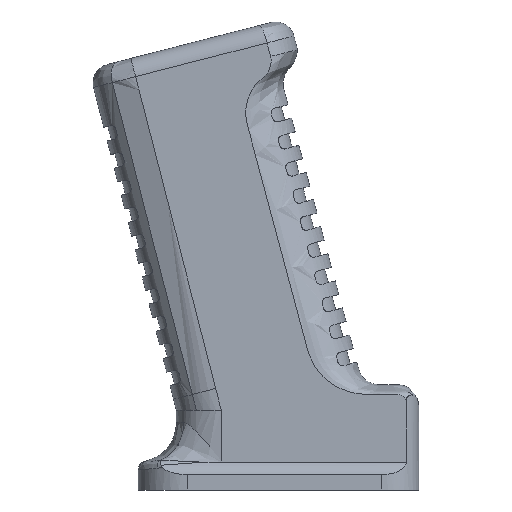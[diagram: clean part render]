
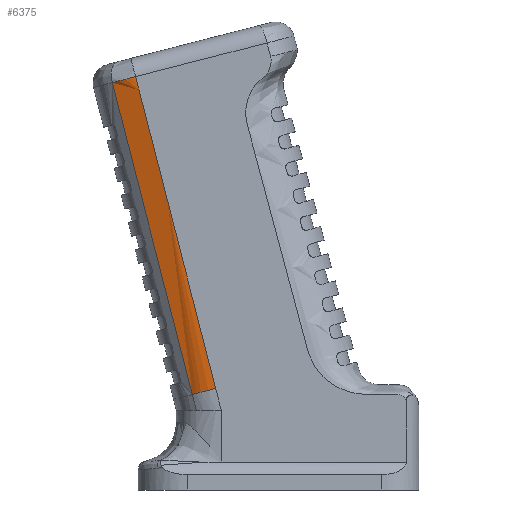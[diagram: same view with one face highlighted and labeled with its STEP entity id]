
A CAD part, front view. The second image highlights one B-rep face of the part: STEP entity #6375.
In plain terms, the highlighted free-form (B-spline) face has degree [3, 1] with [8, 2] control points.
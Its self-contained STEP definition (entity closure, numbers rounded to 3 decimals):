
#403=LINE('',#13296,#897);
#419=LINE('',#13652,#913);
#420=LINE('',#13654,#914);
#421=LINE('',#13656,#915);
#422=LINE('',#13658,#916);
#423=LINE('',#13660,#917);
#897=VECTOR('',#7216,10.);
#913=VECTOR('',#7262,10.);
#914=VECTOR('',#7263,10.);
#915=VECTOR('',#7264,10.);
#916=VECTOR('',#7265,10.);
#917=VECTOR('',#7266,10.);
#1528=FACE_OUTER_BOUND('',#1881,.T.);
#1881=EDGE_LOOP('',(#5424,#5425,#5426,#5427,#5428,#5429,#5430,#5431));
#2388=B_SPLINE_CURVE_WITH_KNOTS('',3,(#18486,#18487,#18488,#18489,#18490,
#18491),.UNSPECIFIED.,.F.,.F.,(4,2,4),(0.,0.025,0.321),
 .UNSPECIFIED.);
#2390=B_SPLINE_CURVE_WITH_KNOTS('',3,(#18559,#18560,#18561,#18562,#18563,
#18564,#18565,#18566,#18567,#18568),.UNSPECIFIED.,.F.,.F.,(4,3,3,4),(-1.549,
-1.43,-1.311,-1.28),.UNSPECIFIED.);
#2753=VERTEX_POINT('',#13281);
#2754=VERTEX_POINT('',#13295);
#2771=VERTEX_POINT('',#13649);
#2772=VERTEX_POINT('',#13651);
#2773=VERTEX_POINT('',#13653);
#2774=VERTEX_POINT('',#13655);
#2775=VERTEX_POINT('',#13657);
#2776=VERTEX_POINT('',#13659);
#3511=EDGE_CURVE('',#2753,#2754,#403,.T.);
#3546=EDGE_CURVE('',#2772,#2771,#419,.T.);
#3547=EDGE_CURVE('',#2773,#2772,#420,.T.);
#3548=EDGE_CURVE('',#2774,#2773,#421,.T.);
#3549=EDGE_CURVE('',#2774,#2775,#422,.T.);
#3550=EDGE_CURVE('',#2775,#2776,#423,.T.);
#3847=EDGE_CURVE('',#2754,#2771,#2388,.T.);
#3865=EDGE_CURVE('',#2776,#2753,#2390,.T.);
#5424=ORIENTED_EDGE('',*,*,#3847,.F.);
#5425=ORIENTED_EDGE('',*,*,#3511,.F.);
#5426=ORIENTED_EDGE('',*,*,#3865,.F.);
#5427=ORIENTED_EDGE('',*,*,#3550,.F.);
#5428=ORIENTED_EDGE('',*,*,#3549,.F.);
#5429=ORIENTED_EDGE('',*,*,#3548,.T.);
#5430=ORIENTED_EDGE('',*,*,#3547,.T.);
#5431=ORIENTED_EDGE('',*,*,#3546,.T.);
#6146=B_SPLINE_SURFACE_WITH_KNOTS('',3,1,((#18543,#18544),(#18545,#18546),
(#18547,#18548),(#18549,#18550),(#18551,#18552),(#18553,#18554),(#18555,
#18556),(#18557,#18558)),.UNSPECIFIED.,.F.,.F.,.F.,(4,2,2,4),(2,2),(1.28,
1.311,1.43,1.549),(0.,7.283),
 .UNSPECIFIED.);
#6375=ADVANCED_FACE('',(#1528),#6146,.T.);
#7216=DIRECTION('',(-0.249,0.,0.969));
#7262=DIRECTION('',(-0.249,0.,0.969));
#7263=DIRECTION('',(-0.249,0.,0.969));
#7264=DIRECTION('',(-0.249,0.,0.969));
#7265=DIRECTION('',(0.249,0.,-0.969));
#7266=DIRECTION('',(0.249,0.,-0.969));
#13281=CARTESIAN_POINT('',(-48.462,-93.535,-93.587));
#13295=CARTESIAN_POINT('',(-65.571,-93.535,-26.913));
#13296=CARTESIAN_POINT('',(-48.462,-93.535,-93.587));
#13649=CARTESIAN_POINT('',(-60.572,-95.182,-25.631));
#13651=CARTESIAN_POINT('',(-60.075,-95.182,-27.568));
#13652=CARTESIAN_POINT('',(-43.463,-95.182,-92.304));
#13653=CARTESIAN_POINT('',(-59.827,-95.182,-28.536));
#13654=CARTESIAN_POINT('',(-59.827,-95.182,-28.536));
#13655=CARTESIAN_POINT('',(-55.411,-95.182,-45.743));
#13656=CARTESIAN_POINT('',(-55.138,-95.182,-46.804));
#13657=CARTESIAN_POINT('',(-53.819,-95.182,-51.944));
#13658=CARTESIAN_POINT('',(-55.139,-95.182,-46.804));
#13659=CARTESIAN_POINT('',(-43.463,-95.182,-92.304));
#13660=CARTESIAN_POINT('',(-46.916,-95.182,-78.831));
#18486=CARTESIAN_POINT('Ctrl Pts',(-65.571,-93.535,-26.913));
#18487=CARTESIAN_POINT('Ctrl Pts',(-65.454,-93.617,
-26.883));
#18488=CARTESIAN_POINT('Ctrl Pts',(-65.334,-93.696,
-26.853));
#18489=CARTESIAN_POINT('Ctrl Pts',(-63.805,-94.653,
-26.46));
#18490=CARTESIAN_POINT('Ctrl Pts',(-62.236,-95.139,-26.057));
#18491=CARTESIAN_POINT('Ctrl Pts',(-60.572,-95.179,
-25.631));
#18543=CARTESIAN_POINT('Ctrl Pts',(-48.462,-93.535,
-93.587));
#18544=CARTESIAN_POINT('Ctrl Pts',(-66.566,-93.535,
-23.039));
#18545=CARTESIAN_POINT('Ctrl Pts',(-48.292,-93.653,-93.544));
#18546=CARTESIAN_POINT('Ctrl Pts',(-66.396,-93.653,
-22.995));
#18547=CARTESIAN_POINT('Ctrl Pts',(-48.118,-93.766,-93.499));
#18548=CARTESIAN_POINT('Ctrl Pts',(-66.222,-93.766,-22.951));
#18549=CARTESIAN_POINT('Ctrl Pts',(-47.263,-94.278,
-93.28));
#18550=CARTESIAN_POINT('Ctrl Pts',(-65.367,-94.278,
-22.731));
#18551=CARTESIAN_POINT('Ctrl Pts',(-46.535,-94.596,
-93.093));
#18552=CARTESIAN_POINT('Ctrl Pts',(-64.639,-94.596,
-22.545));
#18553=CARTESIAN_POINT('Ctrl Pts',(-45.027,-95.037,
-92.706));
#18554=CARTESIAN_POINT('Ctrl Pts',(-63.131,-95.037,
-22.157));
#18555=CARTESIAN_POINT('Ctrl Pts',(-44.247,-95.16,
-92.505));
#18556=CARTESIAN_POINT('Ctrl Pts',(-62.351,-95.16,
-21.957));
#18557=CARTESIAN_POINT('Ctrl Pts',(-43.463,-95.179,
-92.304));
#18558=CARTESIAN_POINT('Ctrl Pts',(-61.567,-95.179,
-21.756));
#18559=CARTESIAN_POINT('Ctrl Pts',(-43.463,-95.179,
-92.304));
#18560=CARTESIAN_POINT('Ctrl Pts',(-44.247,-95.16,
-92.505));
#18561=CARTESIAN_POINT('Ctrl Pts',(-45.027,-95.037,
-92.706));
#18562=CARTESIAN_POINT('Ctrl Pts',(-45.781,-94.816,
-92.899));
#18563=CARTESIAN_POINT('Ctrl Pts',(-46.535,-94.596,
-93.093));
#18564=CARTESIAN_POINT('Ctrl Pts',(-47.263,-94.278,
-93.28));
#18565=CARTESIAN_POINT('Ctrl Pts',(-47.941,-93.872,
-93.454));
#18566=CARTESIAN_POINT('Ctrl Pts',(-48.118,-93.766,
-93.499));
#18567=CARTESIAN_POINT('Ctrl Pts',(-48.292,-93.653,
-93.544));
#18568=CARTESIAN_POINT('Ctrl Pts',(-48.462,-93.535,
-93.587));
